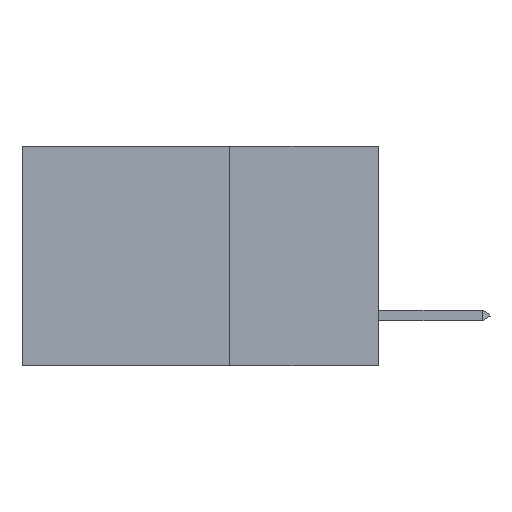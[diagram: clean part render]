
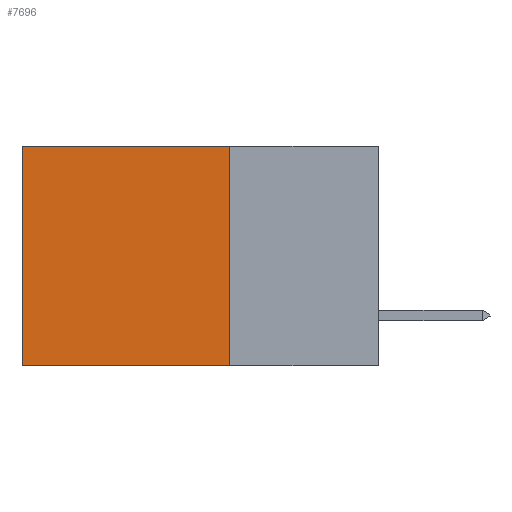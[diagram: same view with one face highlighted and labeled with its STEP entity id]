
A CAD part, left-side view. The second image highlights one B-rep face of the part: STEP entity #7696.
In plain terms, the highlighted planar face has unit normal (-1, 0, 0).
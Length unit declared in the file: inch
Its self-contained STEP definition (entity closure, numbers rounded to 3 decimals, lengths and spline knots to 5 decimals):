
#27 = ORIENTED_EDGE ( 'NONE', *, *, #8845, .F. ) ;
#366 = ORIENTED_EDGE ( 'NONE', *, *, #10244, .F. ) ;
#597 = ORIENTED_EDGE ( 'NONE', *, *, #12824, .T. ) ;
#1018 = PLANE ( 'NONE',  #9503 ) ;
#1836 = CARTESIAN_POINT ( 'NONE',  ( 0.298, 0.6, 0. ) ) ;
#1951 = CARTESIAN_POINT ( 'NONE',  ( 0.298, 0.25, -0.37 ) ) ;
#2030 = DIRECTION ( 'NONE',  ( 0., 0., -1. ) ) ;
#2477 = DIRECTION ( 'NONE',  ( 0., 1., 0. ) ) ;
#3403 = VERTEX_POINT ( 'NONE', #8420 ) ;
#3691 = VERTEX_POINT ( 'NONE', #6585 ) ;
#3897 = VERTEX_POINT ( 'NONE', #13486 ) ;
#3939 = VECTOR ( 'NONE', #2030, 39.37008 ) ;
#5192 = EDGE_LOOP ( 'NONE', ( #13023, #27, #366, #597 ) ) ;
#6466 = CARTESIAN_POINT ( 'NONE',  ( 0.298, 0.25, 0. ) ) ;
#6585 = CARTESIAN_POINT ( 'NONE',  ( 0.298, 0.6, -0.37 ) ) ;
#6934 = VECTOR ( 'NONE', #2477, 39.37008 ) ;
#6959 = CARTESIAN_POINT ( 'NONE',  ( 0.298, 0.6, 0. ) ) ;
#6971 = VECTOR ( 'NONE', #7084, 39.37008 ) ;
#7000 = FACE_OUTER_BOUND ( 'NONE', #5192, .T. ) ;
#7084 = DIRECTION ( 'NONE',  ( 0., 0., -1. ) ) ;
#7677 = LINE ( 'NONE', #13498, #3939 ) ;
#7696 = ADVANCED_FACE ( 'NONE', ( #7000 ), #1018, .F. ) ;
#8135 = LINE ( 'NONE', #1836, #6971 ) ;
#8347 = DIRECTION ( 'NONE',  ( 1., 0., 0. ) ) ;
#8420 = CARTESIAN_POINT ( 'NONE',  ( 0.298, 0.25, 0. ) ) ;
#8557 = EDGE_CURVE ( 'NONE', #10749, #3691, #8135, .T. ) ;
#8845 = EDGE_CURVE ( 'NONE', #3897, #3691, #13073, .T. ) ;
#9359 = DIRECTION ( 'NONE',  ( 0., 0., -1. ) ) ;
#9429 = DIRECTION ( 'NONE',  ( 0., 1., 0. ) ) ;
#9503 = AXIS2_PLACEMENT_3D ( 'NONE', #12492, #8347, #9359 ) ;
#9724 = LINE ( 'NONE', #6466, #6934 ) ;
#10244 = EDGE_CURVE ( 'NONE', #3403, #3897, #7677, .T. ) ;
#10749 = VERTEX_POINT ( 'NONE', #6959 ) ;
#12492 = CARTESIAN_POINT ( 'NONE',  ( 0.298, 0.25, 0. ) ) ;
#12824 = EDGE_CURVE ( 'NONE', #3403, #10749, #9724, .T. ) ;
#13023 = ORIENTED_EDGE ( 'NONE', *, *, #8557, .T. ) ;
#13073 = LINE ( 'NONE', #1951, #13539 ) ;
#13486 = CARTESIAN_POINT ( 'NONE',  ( 0.298, 0.25, -0.37 ) ) ;
#13498 = CARTESIAN_POINT ( 'NONE',  ( 0.298, 0.25, 0. ) ) ;
#13539 = VECTOR ( 'NONE', #9429, 39.37008 ) ;
